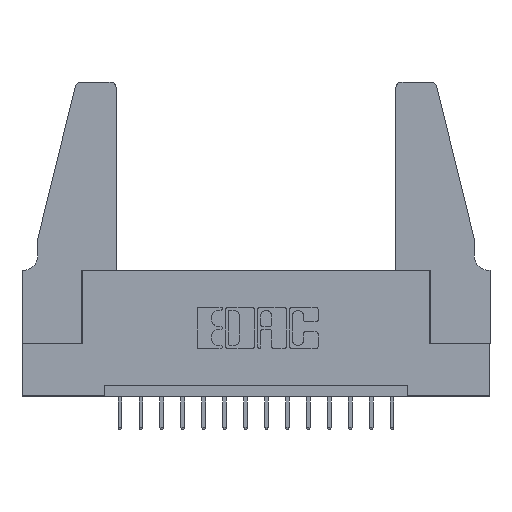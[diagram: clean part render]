
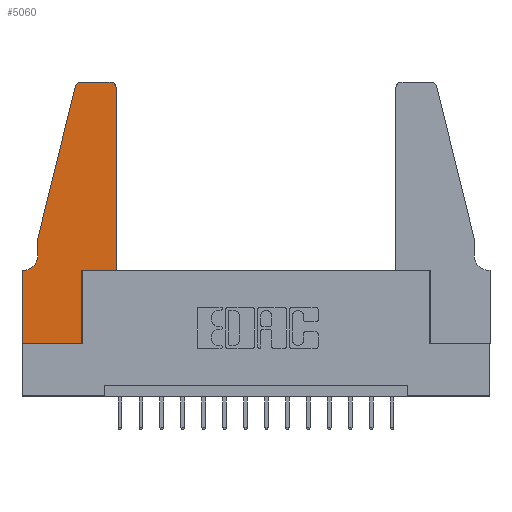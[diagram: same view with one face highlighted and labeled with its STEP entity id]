
A CAD part, top view. The second image highlights one B-rep face of the part: STEP entity #5060.
In plain terms, the highlighted planar face has unit normal (0, 0, 1).
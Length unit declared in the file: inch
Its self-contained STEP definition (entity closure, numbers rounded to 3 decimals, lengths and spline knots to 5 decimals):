
#70 = EDGE_CURVE ( 'NONE', #4191, #9565, #8203, .T. ) ;
#127 = CARTESIAN_POINT ( 'NONE',  ( 0.0755, 0.5, 0.37 ) ) ;
#339 = EDGE_CURVE ( 'NONE', #8638, #7640, #8188, .T. ) ;
#364 = EDGE_CURVE ( 'NONE', #8548, #5042, #12177, .T. ) ;
#534 = CARTESIAN_POINT ( 'NONE',  ( 0.25487, 1.22718, 0.37 ) ) ;
#1106 = CARTESIAN_POINT ( 'NONE',  ( 0.4505, 1.22, 0.37 ) ) ;
#1193 = ORIENTED_EDGE ( 'NONE', *, *, #8434, .T. ) ;
#1310 = CIRCLE ( 'NONE', #15047, 0.03 ) ;
#1686 = FACE_OUTER_BOUND ( 'NONE', #15727, .T. ) ;
#1762 = DIRECTION ( 'NONE',  ( 0., 1., 0. ) ) ;
#1788 = VECTOR ( 'NONE', #11057, 39.37008 ) ;
#1935 = LINE ( 'NONE', #7707, #15128 ) ;
#2018 = EDGE_CURVE ( 'NONE', #3711, #8638, #1935, .T. ) ;
#2161 = VECTOR ( 'NONE', #1762, 39.37008 ) ;
#2754 = DIRECTION ( 'NONE',  ( 1., 0., 0. ) ) ;
#2875 = VERTEX_POINT ( 'NONE', #5241 ) ;
#3056 = CARTESIAN_POINT ( 'NONE',  ( 0.0055, 0.42, 0.37 ) ) ;
#3459 = DIRECTION ( 'NONE',  ( 0., 0., 1. ) ) ;
#3711 = VERTEX_POINT ( 'NONE', #14854 ) ;
#3751 = VECTOR ( 'NONE', #11355, 39.37008 ) ;
#4014 = DIRECTION ( 'NONE',  ( 0., -1., 0. ) ) ;
#4191 = VERTEX_POINT ( 'NONE', #534 ) ;
#4552 = ORIENTED_EDGE ( 'NONE', *, *, #8159, .T. ) ;
#4657 = ORIENTED_EDGE ( 'NONE', *, *, #11426, .T. ) ;
#4844 = EDGE_CURVE ( 'NONE', #2875, #4191, #1310, .T. ) ;
#5032 = DIRECTION ( 'NONE',  ( 0., -1., 0. ) ) ;
#5042 = VERTEX_POINT ( 'NONE', #5538 ) ;
#5060 = ADVANCED_FACE ( 'NONE', ( #1686 ), #14646, .T. ) ;
#5168 = DIRECTION ( 'NONE',  ( 0., 0., 1. ) ) ;
#5241 = CARTESIAN_POINT ( 'NONE',  ( 0.284, 1.25, 0.37 ) ) ;
#5284 = ORIENTED_EDGE ( 'NONE', *, *, #364, .T. ) ;
#5304 = CARTESIAN_POINT ( 'NONE',  ( 0.284, 1.22, 0.37 ) ) ;
#5507 = ORIENTED_EDGE ( 'NONE', *, *, #16361, .T. ) ;
#5538 = CARTESIAN_POINT ( 'NONE',  ( 0.4505, 0.35, 0.37 ) ) ;
#5541 = ORIENTED_EDGE ( 'NONE', *, *, #4844, .T. ) ;
#5958 = EDGE_CURVE ( 'NONE', #9565, #14958, #8248, .T. ) ;
#6018 = DIRECTION ( 'NONE',  ( -1., 0., 0. ) ) ;
#6062 = ORIENTED_EDGE ( 'NONE', *, *, #15380, .T. ) ;
#6468 = DIRECTION ( 'NONE',  ( -1., 0., 0. ) ) ;
#6598 = DIRECTION ( 'NONE',  ( 1., 0., 0. ) ) ;
#6671 = ORIENTED_EDGE ( 'NONE', *, *, #70, .T. ) ;
#7229 = CARTESIAN_POINT ( 'NONE',  ( 0.4505, 0.35, 0.37 ) ) ;
#7377 = CARTESIAN_POINT ( 'NONE',  ( 0., 0.35, 0.37 ) ) ;
#7483 = ORIENTED_EDGE ( 'NONE', *, *, #12993, .T. ) ;
#7541 = DIRECTION ( 'NONE',  ( 0., 1., 0. ) ) ;
#7569 = CARTESIAN_POINT ( 'NONE',  ( 0.4205, 1.25, 0.37 ) ) ;
#7577 = LINE ( 'NONE', #9417, #2161 ) ;
#7640 = VERTEX_POINT ( 'NONE', #7666 ) ;
#7666 = CARTESIAN_POINT ( 'NONE',  ( 0.2865, 0., 0.37 ) ) ;
#7707 = CARTESIAN_POINT ( 'NONE',  ( 0., 0., 0.37 ) ) ;
#7775 = LINE ( 'NONE', #11890, #3751 ) ;
#7894 = CARTESIAN_POINT ( 'NONE',  ( 0.0755, 0.5, 0.37 ) ) ;
#8159 = EDGE_CURVE ( 'NONE', #10440, #3711, #7775, .T. ) ;
#8188 = LINE ( 'NONE', #16013, #10173 ) ;
#8203 = LINE ( 'NONE', #13593, #12784 ) ;
#8248 = LINE ( 'NONE', #127, #15042 ) ;
#8434 = EDGE_CURVE ( 'NONE', #14958, #10440, #11337, .T. ) ;
#8529 = DIRECTION ( 'NONE',  ( -0.239, -0.971, 0. ) ) ;
#8548 = VERTEX_POINT ( 'NONE', #14863 ) ;
#8597 = CARTESIAN_POINT ( 'NONE',  ( 0.2605, 1.25, 0.37 ) ) ;
#8638 = VERTEX_POINT ( 'NONE', #13828 ) ;
#9144 = CARTESIAN_POINT ( 'NONE',  ( 0.4205, 1.22, 0.37 ) ) ;
#9417 = CARTESIAN_POINT ( 'NONE',  ( 0.2865, 0.35, 0.37 ) ) ;
#9565 = VERTEX_POINT ( 'NONE', #7894 ) ;
#9702 = CARTESIAN_POINT ( 'NONE',  ( 0.0055, 0.35, 0.37 ) ) ;
#9711 = LINE ( 'NONE', #8597, #13910 ) ;
#10173 = VECTOR ( 'NONE', #10900, 39.37008 ) ;
#10440 = VERTEX_POINT ( 'NONE', #9702 ) ;
#10601 = VERTEX_POINT ( 'NONE', #1106 ) ;
#10900 = DIRECTION ( 'NONE',  ( 1., 0., 0. ) ) ;
#11057 = DIRECTION ( 'NONE',  ( 1., 0., 0. ) ) ;
#11092 = VERTEX_POINT ( 'NONE', #7569 ) ;
#11337 = CIRCLE ( 'NONE', #13151, 0.07 ) ;
#11355 = DIRECTION ( 'NONE',  ( -1., 0., 0. ) ) ;
#11396 = CARTESIAN_POINT ( 'NONE',  ( 0.0755, 0.42, 0.37 ) ) ;
#11426 = EDGE_CURVE ( 'NONE', #7640, #8548, #7577, .T. ) ;
#11430 = CARTESIAN_POINT ( 'NONE',  ( 0.4505, 0.35, 0.37 ) ) ;
#11890 = CARTESIAN_POINT ( 'NONE',  ( 0.0755, 0.35, 0.37 ) ) ;
#11963 = ORIENTED_EDGE ( 'NONE', *, *, #2018, .T. ) ;
#11994 = DIRECTION ( 'NONE',  ( 0., 0., -1. ) ) ;
#12177 = LINE ( 'NONE', #7229, #1788 ) ;
#12631 = LINE ( 'NONE', #11430, #16254 ) ;
#12784 = VECTOR ( 'NONE', #8529, 39.37008 ) ;
#12993 = EDGE_CURVE ( 'NONE', #11092, #2875, #9711, .T. ) ;
#13151 = AXIS2_PLACEMENT_3D ( 'NONE', #3056, #11994, #6018 ) ;
#13593 = CARTESIAN_POINT ( 'NONE',  ( 0.0755, 0.5, 0.37 ) ) ;
#13828 = CARTESIAN_POINT ( 'NONE',  ( 0., 0., 0.37 ) ) ;
#13910 = VECTOR ( 'NONE', #6468, 39.37008 ) ;
#14241 = DIRECTION ( 'NONE',  ( 0., 0., 1. ) ) ;
#14408 = CIRCLE ( 'NONE', #14716, 0.03 ) ;
#14411 = ORIENTED_EDGE ( 'NONE', *, *, #339, .T. ) ;
#14646 = PLANE ( 'NONE',  #15813 ) ;
#14716 = AXIS2_PLACEMENT_3D ( 'NONE', #9144, #5168, #2754 ) ;
#14854 = CARTESIAN_POINT ( 'NONE',  ( 0., 0.35, 0.37 ) ) ;
#14863 = CARTESIAN_POINT ( 'NONE',  ( 0.2865, 0.35, 0.37 ) ) ;
#14958 = VERTEX_POINT ( 'NONE', #11396 ) ;
#15042 = VECTOR ( 'NONE', #4014, 39.37008 ) ;
#15047 = AXIS2_PLACEMENT_3D ( 'NONE', #5304, #14241, #6598 ) ;
#15128 = VECTOR ( 'NONE', #5032, 39.37008 ) ;
#15331 = ORIENTED_EDGE ( 'NONE', *, *, #5958, .T. ) ;
#15380 = EDGE_CURVE ( 'NONE', #5042, #10601, #12631, .T. ) ;
#15693 = DIRECTION ( 'NONE',  ( 1., 0., 0. ) ) ;
#15727 = EDGE_LOOP ( 'NONE', ( #7483, #5541, #6671, #15331, #1193, #4552, #11963, #14411, #4657, #5284, #6062, #5507 ) ) ;
#15813 = AXIS2_PLACEMENT_3D ( 'NONE', #7377, #3459, #15693 ) ;
#16013 = CARTESIAN_POINT ( 'NONE',  ( 0., 0., 0.37 ) ) ;
#16254 = VECTOR ( 'NONE', #7541, 39.37008 ) ;
#16361 = EDGE_CURVE ( 'NONE', #10601, #11092, #14408, .T. ) ;
